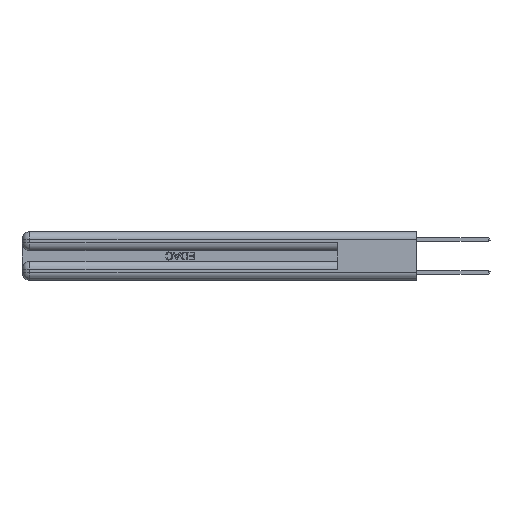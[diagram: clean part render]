
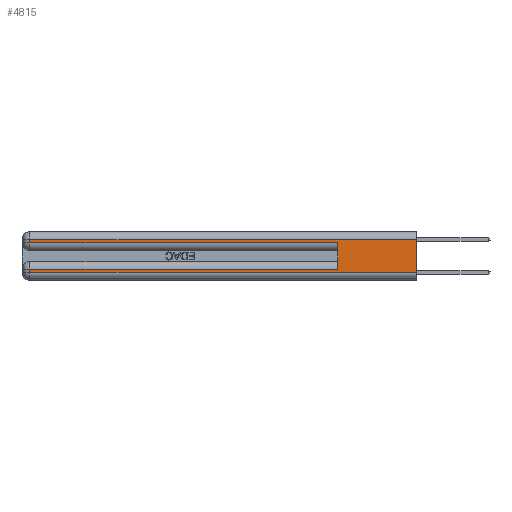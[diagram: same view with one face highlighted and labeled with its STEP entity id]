
A CAD part, left-side view. The second image highlights one B-rep face of the part: STEP entity #4815.
In plain terms, the highlighted planar face has unit normal (-1, 0, 0).
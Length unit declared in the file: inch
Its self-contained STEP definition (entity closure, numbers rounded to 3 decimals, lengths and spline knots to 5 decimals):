
#661 = EDGE_CURVE ( 'NONE', #35477, #35776, #26154, .T. ) ;
#2206 = CARTESIAN_POINT ( 'NONE',  ( 0., 0., 0.37 ) ) ;
#2858 = ORIENTED_EDGE ( 'NONE', *, *, #34734, .F. ) ;
#3325 = VERTEX_POINT ( 'NONE', #6690 ) ;
#4168 = CARTESIAN_POINT ( 'NONE',  ( 0., 2.94, 0.085 ) ) ;
#4449 = DIRECTION ( 'NONE',  ( 0., 0., -1. ) ) ;
#4815 = ADVANCED_FACE ( 'NONE', ( #18937 ), #33255, .F. ) ;
#5174 = LINE ( 'NONE', #22446, #8193 ) ;
#5844 = EDGE_CURVE ( 'NONE', #13237, #3325, #34557, .T. ) ;
#5952 = CARTESIAN_POINT ( 'NONE',  ( 0., 0., 0.285 ) ) ;
#6690 = CARTESIAN_POINT ( 'NONE',  ( 0., 0.6, 0.285 ) ) ;
#7392 = EDGE_CURVE ( 'NONE', #20525, #7756, #5174, .T. ) ;
#7756 = VERTEX_POINT ( 'NONE', #36528 ) ;
#8193 = VECTOR ( 'NONE', #19471, 39.37008 ) ;
#8927 = LINE ( 'NONE', #28979, #34004 ) ;
#10061 = VERTEX_POINT ( 'NONE', #13335 ) ;
#12374 = CARTESIAN_POINT ( 'NONE',  ( 0., 0., 0.31 ) ) ;
#12749 = ORIENTED_EDGE ( 'NONE', *, *, #661, .T. ) ;
#13202 = EDGE_LOOP ( 'NONE', ( #26829, #25277, #27975, #26911, #2858, #15176, #12749, #24809 ) ) ;
#13237 = VERTEX_POINT ( 'NONE', #20503 ) ;
#13335 = CARTESIAN_POINT ( 'NONE',  ( 0., 0.6, 0.085 ) ) ;
#14193 = EDGE_CURVE ( 'NONE', #10061, #35477, #19285, .T. ) ;
#14858 = DIRECTION ( 'NONE',  ( 0., 0., 1. ) ) ;
#15176 = ORIENTED_EDGE ( 'NONE', *, *, #14193, .T. ) ;
#16348 = EDGE_CURVE ( 'NONE', #35776, #7756, #19940, .T. ) ;
#16990 = VECTOR ( 'NONE', #20059, 39.37008 ) ;
#18937 = FACE_OUTER_BOUND ( 'NONE', #13202, .T. ) ;
#19285 = LINE ( 'NONE', #22257, #32149 ) ;
#19401 = DIRECTION ( 'NONE',  ( 0., 1., 0. ) ) ;
#19471 = DIRECTION ( 'NONE',  ( 0., 0., -1. ) ) ;
#19940 = LINE ( 'NONE', #34083, #33361 ) ;
#20059 = DIRECTION ( 'NONE',  ( 0., -1., 0. ) ) ;
#20503 = CARTESIAN_POINT ( 'NONE',  ( 0., 2.94, 0.285 ) ) ;
#20525 = VERTEX_POINT ( 'NONE', #12374 ) ;
#20543 = VERTEX_POINT ( 'NONE', #20722 ) ;
#20722 = CARTESIAN_POINT ( 'NONE',  ( 0., 2.94, 0.31 ) ) ;
#20757 = VECTOR ( 'NONE', #19401, 39.37008 ) ;
#22253 = EDGE_CURVE ( 'NONE', #20543, #13237, #29221, .T. ) ;
#22257 = CARTESIAN_POINT ( 'NONE',  ( 0., 0., 0.085 ) ) ;
#22446 = CARTESIAN_POINT ( 'NONE',  ( 0., 0., 0.37 ) ) ;
#23100 = CARTESIAN_POINT ( 'NONE',  ( 0., 2.94, 0.37 ) ) ;
#23915 = DIRECTION ( 'NONE',  ( 0., 0., -1. ) ) ;
#24809 = ORIENTED_EDGE ( 'NONE', *, *, #16348, .T. ) ;
#25277 = ORIENTED_EDGE ( 'NONE', *, *, #32664, .T. ) ;
#25838 = CARTESIAN_POINT ( 'NONE',  ( 0., 2.94, 0.06 ) ) ;
#26154 = LINE ( 'NONE', #29131, #27706 ) ;
#26829 = ORIENTED_EDGE ( 'NONE', *, *, #7392, .F. ) ;
#26859 = VECTOR ( 'NONE', #34626, 39.37008 ) ;
#26911 = ORIENTED_EDGE ( 'NONE', *, *, #5844, .T. ) ;
#27706 = VECTOR ( 'NONE', #23915, 39.37008 ) ;
#27975 = ORIENTED_EDGE ( 'NONE', *, *, #22253, .T. ) ;
#28979 = CARTESIAN_POINT ( 'NONE',  ( 0., 0.6, 0.145 ) ) ;
#29131 = CARTESIAN_POINT ( 'NONE',  ( 0., 2.94, 0.37 ) ) ;
#29221 = LINE ( 'NONE', #23100, #26859 ) ;
#31205 = AXIS2_PLACEMENT_3D ( 'NONE', #2206, #36213, #4449 ) ;
#32149 = VECTOR ( 'NONE', #33429, 39.37008 ) ;
#32664 = EDGE_CURVE ( 'NONE', #20525, #20543, #33367, .T. ) ;
#33255 = PLANE ( 'NONE',  #31205 ) ;
#33361 = VECTOR ( 'NONE', #34449, 39.37008 ) ;
#33367 = LINE ( 'NONE', #33546, #20757 ) ;
#33429 = DIRECTION ( 'NONE',  ( 0., 1., 0. ) ) ;
#33546 = CARTESIAN_POINT ( 'NONE',  ( 0., 0., 0.31 ) ) ;
#34004 = VECTOR ( 'NONE', #14858, 39.37008 ) ;
#34083 = CARTESIAN_POINT ( 'NONE',  ( 0., 0., 0.06 ) ) ;
#34449 = DIRECTION ( 'NONE',  ( 0., -1., 0. ) ) ;
#34557 = LINE ( 'NONE', #5952, #16990 ) ;
#34626 = DIRECTION ( 'NONE',  ( 0., 0., -1. ) ) ;
#34734 = EDGE_CURVE ( 'NONE', #10061, #3325, #8927, .T. ) ;
#35477 = VERTEX_POINT ( 'NONE', #4168 ) ;
#35776 = VERTEX_POINT ( 'NONE', #25838 ) ;
#36213 = DIRECTION ( 'NONE',  ( 1., 0., 0. ) ) ;
#36528 = CARTESIAN_POINT ( 'NONE',  ( 0., 0., 0.06 ) ) ;
